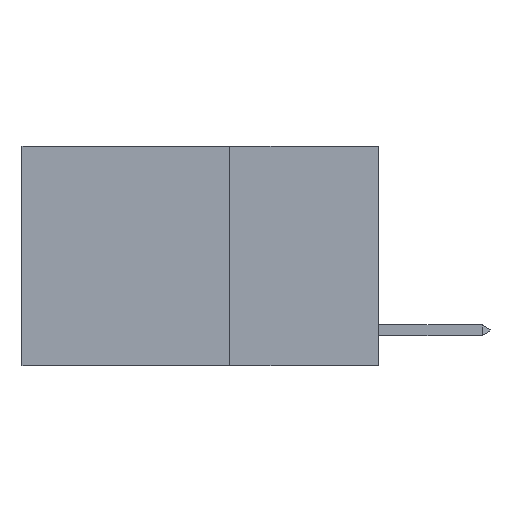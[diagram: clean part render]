
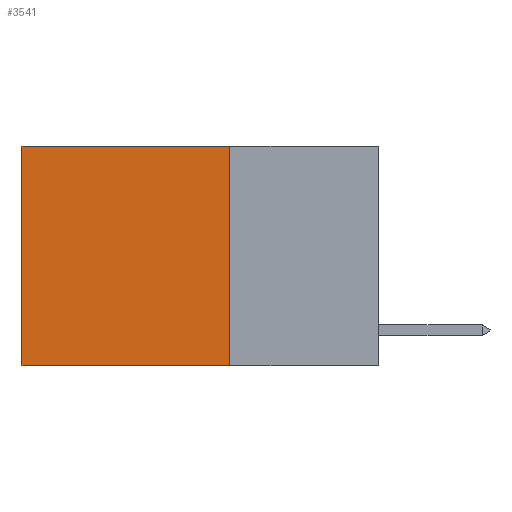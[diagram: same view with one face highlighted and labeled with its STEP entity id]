
A CAD part, left-side view. The second image highlights one B-rep face of the part: STEP entity #3541.
In plain terms, the highlighted planar face has unit normal (-1, 0, 0).
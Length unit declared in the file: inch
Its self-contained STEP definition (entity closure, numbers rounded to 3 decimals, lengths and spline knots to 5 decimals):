
#1024 = ORIENTED_EDGE ( 'NONE', *, *, #10294, .F. ) ;
#2105 = DIRECTION ( 'NONE',  ( 0., 0., -1. ) ) ;
#2827 = LINE ( 'NONE', #18124, #15842 ) ;
#3353 = EDGE_CURVE ( 'NONE', #11659, #19016, #2827, .T. ) ;
#3541 = ADVANCED_FACE ( 'NONE', ( #8568 ), #19220, .F. ) ;
#4334 = DIRECTION ( 'NONE',  ( 0., 0., -1. ) ) ;
#4587 = VECTOR ( 'NONE', #15370, 39.37008 ) ;
#5003 = CARTESIAN_POINT ( 'NONE',  ( 0.2625, 0.25, 0. ) ) ;
#5760 = CARTESIAN_POINT ( 'NONE',  ( 0.2625, 0.6, 0. ) ) ;
#5903 = AXIS2_PLACEMENT_3D ( 'NONE', #14799, #14603, #2105 ) ;
#6038 = VECTOR ( 'NONE', #4334, 39.37008 ) ;
#8568 = FACE_OUTER_BOUND ( 'NONE', #17492, .T. ) ;
#9525 = ORIENTED_EDGE ( 'NONE', *, *, #9757, .T. ) ;
#9757 = EDGE_CURVE ( 'NONE', #11659, #16990, #15569, .T. ) ;
#9935 = DIRECTION ( 'NONE',  ( 0., 1., 0. ) ) ;
#9940 = CARTESIAN_POINT ( 'NONE',  ( 0.2625, 0.25, 0. ) ) ;
#10294 = EDGE_CURVE ( 'NONE', #19016, #15454, #18860, .T. ) ;
#10708 = DIRECTION ( 'NONE',  ( 0., 0., -1. ) ) ;
#11659 = VERTEX_POINT ( 'NONE', #9940 ) ;
#13170 = CARTESIAN_POINT ( 'NONE',  ( 0.2625, 0.25, -0.37 ) ) ;
#13239 = LINE ( 'NONE', #5760, #6038 ) ;
#13423 = ORIENTED_EDGE ( 'NONE', *, *, #18606, .T. ) ;
#13631 = ORIENTED_EDGE ( 'NONE', *, *, #3353, .F. ) ;
#13670 = CARTESIAN_POINT ( 'NONE',  ( 0.2625, 0.25, -0.37 ) ) ;
#14603 = DIRECTION ( 'NONE',  ( 1., 0., 0. ) ) ;
#14799 = CARTESIAN_POINT ( 'NONE',  ( 0.2625, 0.25, 0. ) ) ;
#15370 = DIRECTION ( 'NONE',  ( 0., 1., 0. ) ) ;
#15454 = VERTEX_POINT ( 'NONE', #18629 ) ;
#15569 = LINE ( 'NONE', #5003, #4587 ) ;
#15842 = VECTOR ( 'NONE', #10708, 39.37008 ) ;
#16990 = VERTEX_POINT ( 'NONE', #17291 ) ;
#17291 = CARTESIAN_POINT ( 'NONE',  ( 0.2625, 0.6, 0. ) ) ;
#17492 = EDGE_LOOP ( 'NONE', ( #13423, #1024, #13631, #9525 ) ) ;
#18124 = CARTESIAN_POINT ( 'NONE',  ( 0.2625, 0.25, 0. ) ) ;
#18606 = EDGE_CURVE ( 'NONE', #16990, #15454, #13239, .T. ) ;
#18629 = CARTESIAN_POINT ( 'NONE',  ( 0.2625, 0.6, -0.37 ) ) ;
#18860 = LINE ( 'NONE', #13170, #19382 ) ;
#19016 = VERTEX_POINT ( 'NONE', #13670 ) ;
#19220 = PLANE ( 'NONE',  #5903 ) ;
#19382 = VECTOR ( 'NONE', #9935, 39.37008 ) ;
